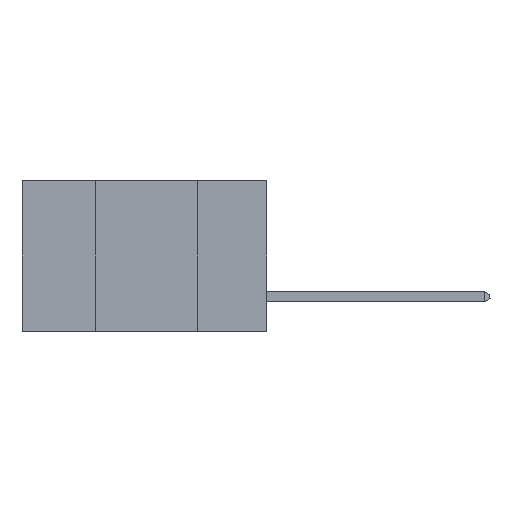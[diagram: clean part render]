
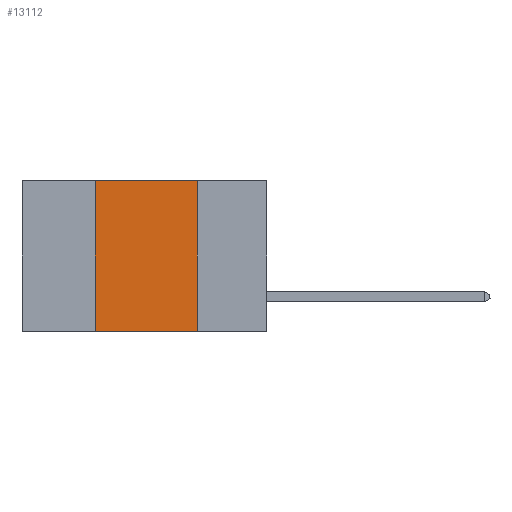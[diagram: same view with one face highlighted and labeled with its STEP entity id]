
A CAD part, left-side view. The second image highlights one B-rep face of the part: STEP entity #13112.
In plain terms, the highlighted planar face has unit normal (-1, 0, 0).
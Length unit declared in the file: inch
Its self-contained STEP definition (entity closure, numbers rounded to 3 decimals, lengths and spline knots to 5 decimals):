
#232 = VERTEX_POINT ( 'NONE', #12223 ) ;
#544 = DIRECTION ( 'NONE',  ( 0., 0., 1. ) ) ;
#778 = DIRECTION ( 'NONE',  ( 1., 0., 0. ) ) ;
#1511 = VECTOR ( 'NONE', #15656, 39.37008 ) ;
#1544 = VERTEX_POINT ( 'NONE', #7738 ) ;
#2724 = ORIENTED_EDGE ( 'NONE', *, *, #7913, .F. ) ;
#3037 = VECTOR ( 'NONE', #544, 39.37008 ) ;
#3065 = CARTESIAN_POINT ( 'NONE',  ( 0., 0.42, 0. ) ) ;
#3313 = ORIENTED_EDGE ( 'NONE', *, *, #12044, .F. ) ;
#3357 = EDGE_CURVE ( 'NONE', #8921, #1544, #6254, .T. ) ;
#4196 = CARTESIAN_POINT ( 'NONE',  ( 0., 0.6, 0. ) ) ;
#4607 = AXIS2_PLACEMENT_3D ( 'NONE', #4196, #778, #5519 ) ;
#5519 = DIRECTION ( 'NONE',  ( 0., 0., -1. ) ) ;
#6227 = CARTESIAN_POINT ( 'NONE',  ( 0., 0.6, 0. ) ) ;
#6254 = LINE ( 'NONE', #3065, #3037 ) ;
#6356 = CARTESIAN_POINT ( 'NONE',  ( 0., 0.6, -0.37 ) ) ;
#6475 = CARTESIAN_POINT ( 'NONE',  ( 0., 0.17, 0. ) ) ;
#6746 = ORIENTED_EDGE ( 'NONE', *, *, #10793, .T. ) ;
#7738 = CARTESIAN_POINT ( 'NONE',  ( 0., 0.42, 0. ) ) ;
#7861 = FACE_OUTER_BOUND ( 'NONE', #15561, .T. ) ;
#7913 = EDGE_CURVE ( 'NONE', #14219, #232, #13052, .T. ) ;
#8921 = VERTEX_POINT ( 'NONE', #12906 ) ;
#9510 = CARTESIAN_POINT ( 'NONE',  ( 0., 0.17, 0. ) ) ;
#9550 = VECTOR ( 'NONE', #14691, 39.37008 ) ;
#10461 = PLANE ( 'NONE',  #4607 ) ;
#10793 = EDGE_CURVE ( 'NONE', #8921, #232, #11112, .T. ) ;
#11068 = LINE ( 'NONE', #6227, #9550 ) ;
#11112 = LINE ( 'NONE', #6356, #15467 ) ;
#11312 = ORIENTED_EDGE ( 'NONE', *, *, #3357, .F. ) ;
#12044 = EDGE_CURVE ( 'NONE', #1544, #14219, #11068, .T. ) ;
#12223 = CARTESIAN_POINT ( 'NONE',  ( 0., 0.17, -0.37 ) ) ;
#12906 = CARTESIAN_POINT ( 'NONE',  ( 0., 0.42, -0.37 ) ) ;
#13052 = LINE ( 'NONE', #9510, #1511 ) ;
#13112 = ADVANCED_FACE ( 'NONE', ( #7861 ), #10461, .F. ) ;
#13645 = DIRECTION ( 'NONE',  ( 0., -1., 0. ) ) ;
#14219 = VERTEX_POINT ( 'NONE', #6475 ) ;
#14691 = DIRECTION ( 'NONE',  ( 0., -1., 0. ) ) ;
#15467 = VECTOR ( 'NONE', #13645, 39.37008 ) ;
#15561 = EDGE_LOOP ( 'NONE', ( #2724, #3313, #11312, #6746 ) ) ;
#15656 = DIRECTION ( 'NONE',  ( 0., 0., -1. ) ) ;
